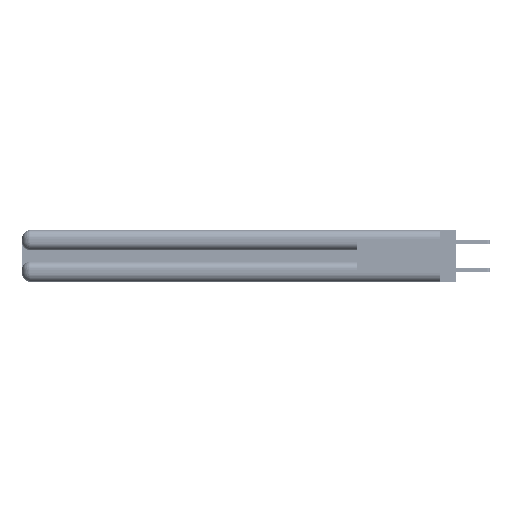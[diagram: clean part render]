
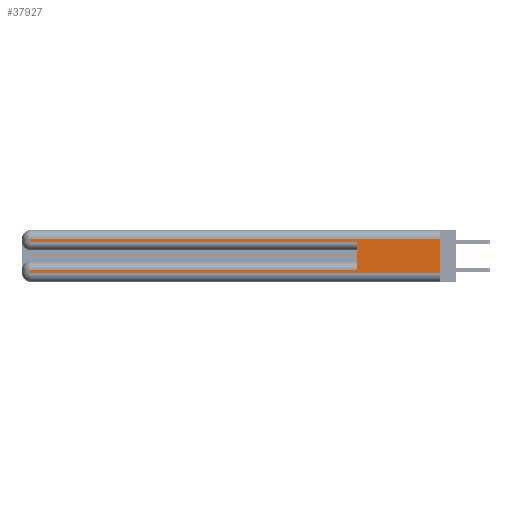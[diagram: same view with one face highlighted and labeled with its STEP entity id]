
A CAD part, left-side view. The second image highlights one B-rep face of the part: STEP entity #37927.
In plain terms, the highlighted planar face has unit normal (-1, 0, 0).
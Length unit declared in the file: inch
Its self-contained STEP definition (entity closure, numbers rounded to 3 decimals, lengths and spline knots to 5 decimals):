
#1482 = VECTOR ( 'NONE', #9272, 39.37008 ) ;
#1740 = VECTOR ( 'NONE', #40676, 39.37008 ) ;
#1750 = CARTESIAN_POINT ( 'NONE',  ( 0., 0., 0.37 ) ) ;
#2334 = LINE ( 'NONE', #22586, #20584 ) ;
#2659 = VECTOR ( 'NONE', #18736, 39.37008 ) ;
#2920 = EDGE_CURVE ( 'NONE', #36948, #11489, #13019, .T. ) ;
#3094 = ORIENTED_EDGE ( 'NONE', *, *, #50283, .T. ) ;
#6210 = DIRECTION ( 'NONE',  ( 1., 0., 0. ) ) ;
#6215 = VERTEX_POINT ( 'NONE', #8320 ) ;
#7498 = LINE ( 'NONE', #49175, #14138 ) ;
#8179 = FACE_OUTER_BOUND ( 'NONE', #17985, .T. ) ;
#8320 = CARTESIAN_POINT ( 'NONE',  ( 0., 0.6, 0.085 ) ) ;
#9272 = DIRECTION ( 'NONE',  ( 0., 0., 1. ) ) ;
#9400 = LINE ( 'NONE', #34789, #41821 ) ;
#9574 = CARTESIAN_POINT ( 'NONE',  ( 0., 2.94, 0.37 ) ) ;
#10704 = EDGE_CURVE ( 'NONE', #6215, #29400, #27121, .T. ) ;
#10800 = CARTESIAN_POINT ( 'NONE',  ( 0., 0., 0.06 ) ) ;
#11262 = CARTESIAN_POINT ( 'NONE',  ( 0., 0.6, 0.285 ) ) ;
#11489 = VERTEX_POINT ( 'NONE', #13937 ) ;
#11749 = EDGE_CURVE ( 'NONE', #32724, #18709, #9400, .T. ) ;
#13019 = LINE ( 'NONE', #10800, #2659 ) ;
#13333 = PLANE ( 'NONE',  #33573 ) ;
#13937 = CARTESIAN_POINT ( 'NONE',  ( 0., 0., 0.06 ) ) ;
#14116 = DIRECTION ( 'NONE',  ( 0., 1., 0. ) ) ;
#14138 = VECTOR ( 'NONE', #14116, 39.37008 ) ;
#14234 = ORIENTED_EDGE ( 'NONE', *, *, #34036, .T. ) ;
#15046 = VERTEX_POINT ( 'NONE', #24723 ) ;
#15245 = ORIENTED_EDGE ( 'NONE', *, *, #48876, .T. ) ;
#17234 = DIRECTION ( 'NONE',  ( 0., 0., -1. ) ) ;
#17844 = ORIENTED_EDGE ( 'NONE', *, *, #2920, .T. ) ;
#17985 = EDGE_LOOP ( 'NONE', ( #25934, #21832, #20643, #14234, #43233, #15245, #3094, #17844 ) ) ;
#17999 = CARTESIAN_POINT ( 'NONE',  ( 0., 0., 0.37 ) ) ;
#18321 = DIRECTION ( 'NONE',  ( 0., -1., 0. ) ) ;
#18709 = VERTEX_POINT ( 'NONE', #38004 ) ;
#18736 = DIRECTION ( 'NONE',  ( 0., -1., 0. ) ) ;
#19218 = EDGE_CURVE ( 'NONE', #18709, #15046, #37867, .T. ) ;
#20340 = EDGE_CURVE ( 'NONE', #32724, #11489, #42499, .T. ) ;
#20584 = VECTOR ( 'NONE', #18321, 39.37008 ) ;
#20643 = ORIENTED_EDGE ( 'NONE', *, *, #19218, .T. ) ;
#21832 = ORIENTED_EDGE ( 'NONE', *, *, #11749, .T. ) ;
#22586 = CARTESIAN_POINT ( 'NONE',  ( 0., 0., 0.285 ) ) ;
#24374 = VERTEX_POINT ( 'NONE', #27128 ) ;
#24723 = CARTESIAN_POINT ( 'NONE',  ( 0., 2.94, 0.285 ) ) ;
#25840 = VECTOR ( 'NONE', #49998, 39.37008 ) ;
#25934 = ORIENTED_EDGE ( 'NONE', *, *, #20340, .F. ) ;
#27121 = LINE ( 'NONE', #36448, #1482 ) ;
#27128 = CARTESIAN_POINT ( 'NONE',  ( 0., 2.94, 0.085 ) ) ;
#29400 = VERTEX_POINT ( 'NONE', #11262 ) ;
#31663 = DIRECTION ( 'NONE',  ( 0., 1., 0. ) ) ;
#32724 = VERTEX_POINT ( 'NONE', #48584 ) ;
#33573 = AXIS2_PLACEMENT_3D ( 'NONE', #1750, #6210, #17234 ) ;
#34036 = EDGE_CURVE ( 'NONE', #15046, #29400, #2334, .T. ) ;
#34789 = CARTESIAN_POINT ( 'NONE',  ( 0., 0., 0.31 ) ) ;
#36448 = CARTESIAN_POINT ( 'NONE',  ( 0., 0.6, 0.145 ) ) ;
#36948 = VERTEX_POINT ( 'NONE', #46621 ) ;
#37867 = LINE ( 'NONE', #9574, #1740 ) ;
#37927 = ADVANCED_FACE ( 'NONE', ( #8179 ), #13333, .F. ) ;
#38004 = CARTESIAN_POINT ( 'NONE',  ( 0., 2.94, 0.31 ) ) ;
#38011 = VECTOR ( 'NONE', #39004, 39.37008 ) ;
#39004 = DIRECTION ( 'NONE',  ( 0., 0., -1. ) ) ;
#40676 = DIRECTION ( 'NONE',  ( 0., 0., -1. ) ) ;
#41821 = VECTOR ( 'NONE', #31663, 39.37008 ) ;
#42499 = LINE ( 'NONE', #17999, #25840 ) ;
#42740 = CARTESIAN_POINT ( 'NONE',  ( 0., 2.94, 0.37 ) ) ;
#43233 = ORIENTED_EDGE ( 'NONE', *, *, #10704, .F. ) ;
#46621 = CARTESIAN_POINT ( 'NONE',  ( 0., 2.94, 0.06 ) ) ;
#47143 = LINE ( 'NONE', #42740, #38011 ) ;
#48584 = CARTESIAN_POINT ( 'NONE',  ( 0., 0., 0.31 ) ) ;
#48876 = EDGE_CURVE ( 'NONE', #6215, #24374, #7498, .T. ) ;
#49175 = CARTESIAN_POINT ( 'NONE',  ( 0., 0., 0.085 ) ) ;
#49998 = DIRECTION ( 'NONE',  ( 0., 0., -1. ) ) ;
#50283 = EDGE_CURVE ( 'NONE', #24374, #36948, #47143, .T. ) ;
